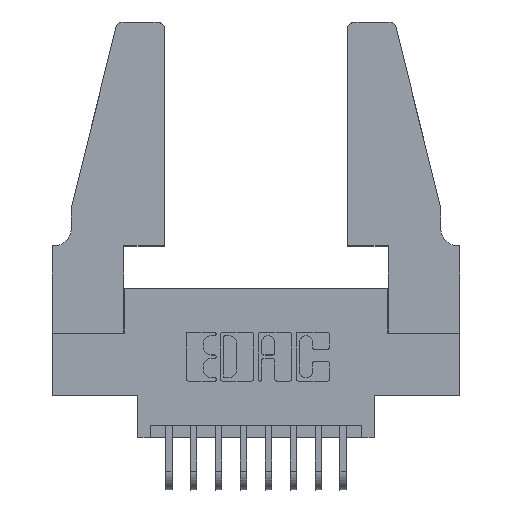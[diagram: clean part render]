
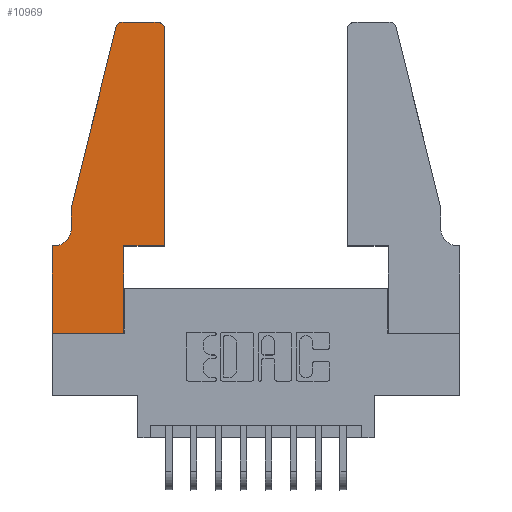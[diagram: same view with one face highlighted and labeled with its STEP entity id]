
A CAD part, top view. The second image highlights one B-rep face of the part: STEP entity #10969.
In plain terms, the highlighted planar face has unit normal (0, 0, 1).
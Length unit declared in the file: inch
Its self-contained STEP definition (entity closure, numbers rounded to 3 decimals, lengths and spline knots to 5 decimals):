
#28 = CARTESIAN_POINT ( 'NONE',  ( 0.25487, 1.22718, 0.37 ) ) ;
#66 = CARTESIAN_POINT ( 'NONE',  ( 0.2865, 0.35, 0.37 ) ) ;
#365 = LINE ( 'NONE', #3650, #8227 ) ;
#693 = VECTOR ( 'NONE', #12470, 39.37008 ) ;
#808 = ORIENTED_EDGE ( 'NONE', *, *, #6925, .T. ) ;
#941 = CARTESIAN_POINT ( 'NONE',  ( 0.4505, 0.35, 0.37 ) ) ;
#954 = ORIENTED_EDGE ( 'NONE', *, *, #7182, .T. ) ;
#988 = CARTESIAN_POINT ( 'NONE',  ( 0.2865, 0.35, 0.37 ) ) ;
#1146 = VERTEX_POINT ( 'NONE', #13948 ) ;
#1562 = ORIENTED_EDGE ( 'NONE', *, *, #14739, .T. ) ;
#1564 = LINE ( 'NONE', #11279, #4241 ) ;
#1579 = LINE ( 'NONE', #7947, #693 ) ;
#1586 = DIRECTION ( 'NONE',  ( 0., 0., 1. ) ) ;
#1688 = CARTESIAN_POINT ( 'NONE',  ( 0.4205, 1.22, 0.37 ) ) ;
#2029 = LINE ( 'NONE', #8240, #6129 ) ;
#2648 = EDGE_CURVE ( 'NONE', #11795, #11288, #12134, .T. ) ;
#2776 = EDGE_CURVE ( 'NONE', #5609, #3500, #8960, .T. ) ;
#3038 = FACE_OUTER_BOUND ( 'NONE', #5361, .T. ) ;
#3050 = DIRECTION ( 'NONE',  ( 0., 0., 1. ) ) ;
#3183 = EDGE_CURVE ( 'NONE', #1146, #6017, #3889, .T. ) ;
#3237 = EDGE_CURVE ( 'NONE', #3848, #1146, #1579, .T. ) ;
#3498 = DIRECTION ( 'NONE',  ( 0., 0., -1. ) ) ;
#3500 = VERTEX_POINT ( 'NONE', #6154 ) ;
#3650 = CARTESIAN_POINT ( 'NONE',  ( 0., 0., 0.37 ) ) ;
#3815 = ORIENTED_EDGE ( 'NONE', *, *, #7220, .T. ) ;
#3848 = VERTEX_POINT ( 'NONE', #3857 ) ;
#3857 = CARTESIAN_POINT ( 'NONE',  ( 0., 0., 0.37 ) ) ;
#3889 = LINE ( 'NONE', #988, #4594 ) ;
#4046 = PLANE ( 'NONE',  #5932 ) ;
#4065 = VERTEX_POINT ( 'NONE', #941 ) ;
#4241 = VECTOR ( 'NONE', #4418, 39.37008 ) ;
#4335 = AXIS2_PLACEMENT_3D ( 'NONE', #9169, #3498, #12606 ) ;
#4418 = DIRECTION ( 'NONE',  ( -1., 0., 0. ) ) ;
#4440 = ORIENTED_EDGE ( 'NONE', *, *, #3183, .T. ) ;
#4594 = VECTOR ( 'NONE', #6827, 39.37008 ) ;
#4680 = AXIS2_PLACEMENT_3D ( 'NONE', #1688, #1586, #14358 ) ;
#4840 = VECTOR ( 'NONE', #13643, 39.37008 ) ;
#5280 = DIRECTION ( 'NONE',  ( 1., 0., 0. ) ) ;
#5361 = EDGE_LOOP ( 'NONE', ( #3815, #8125, #5536, #9611, #8568, #6661, #1562, #12802, #4440, #13207, #954, #808 ) ) ;
#5536 = ORIENTED_EDGE ( 'NONE', *, *, #6741, .T. ) ;
#5609 = VERTEX_POINT ( 'NONE', #10730 ) ;
#5837 = VERTEX_POINT ( 'NONE', #13208 ) ;
#5872 = VECTOR ( 'NONE', #6796, 39.37008 ) ;
#5932 = AXIS2_PLACEMENT_3D ( 'NONE', #7614, #3050, #5280 ) ;
#6017 = VERTEX_POINT ( 'NONE', #66 ) ;
#6129 = VECTOR ( 'NONE', #9478, 39.37008 ) ;
#6154 = CARTESIAN_POINT ( 'NONE',  ( 0.0755, 0.42, 0.37 ) ) ;
#6302 = EDGE_CURVE ( 'NONE', #6017, #4065, #8851, .T. ) ;
#6324 = VECTOR ( 'NONE', #14458, 39.37008 ) ;
#6378 = CARTESIAN_POINT ( 'NONE',  ( 0.0755, 0.35, 0.37 ) ) ;
#6543 = CARTESIAN_POINT ( 'NONE',  ( 0.284, 1.22, 0.37 ) ) ;
#6596 = DIRECTION ( 'NONE',  ( 0., 0., 1. ) ) ;
#6661 = ORIENTED_EDGE ( 'NONE', *, *, #13215, .T. ) ;
#6741 = EDGE_CURVE ( 'NONE', #11288, #5609, #2029, .T. ) ;
#6796 = DIRECTION ( 'NONE',  ( 0., -1., 0. ) ) ;
#6827 = DIRECTION ( 'NONE',  ( 0., 1., 0. ) ) ;
#6925 = EDGE_CURVE ( 'NONE', #10156, #10413, #11331, .T. ) ;
#7182 = EDGE_CURVE ( 'NONE', #4065, #10156, #14001, .T. ) ;
#7220 = EDGE_CURVE ( 'NONE', #10413, #11795, #1564, .T. ) ;
#7614 = CARTESIAN_POINT ( 'NONE',  ( 0., 0.35, 0.37 ) ) ;
#7713 = DIRECTION ( 'NONE',  ( 1., 0., 0. ) ) ;
#7840 = CARTESIAN_POINT ( 'NONE',  ( 0.4505, 0.35, 0.37 ) ) ;
#7947 = CARTESIAN_POINT ( 'NONE',  ( 0., 0., 0.37 ) ) ;
#8125 = ORIENTED_EDGE ( 'NONE', *, *, #2648, .T. ) ;
#8227 = VECTOR ( 'NONE', #9466, 39.37008 ) ;
#8240 = CARTESIAN_POINT ( 'NONE',  ( 0.0755, 0.5, 0.37 ) ) ;
#8548 = VECTOR ( 'NONE', #9728, 39.37008 ) ;
#8568 = ORIENTED_EDGE ( 'NONE', *, *, #11293, .T. ) ;
#8851 = LINE ( 'NONE', #13198, #6324 ) ;
#8960 = LINE ( 'NONE', #10045, #5872 ) ;
#9169 = CARTESIAN_POINT ( 'NONE',  ( 0.0055, 0.42, 0.37 ) ) ;
#9466 = DIRECTION ( 'NONE',  ( 0., -1., 0. ) ) ;
#9478 = DIRECTION ( 'NONE',  ( -0.239, -0.971, 0. ) ) ;
#9611 = ORIENTED_EDGE ( 'NONE', *, *, #2776, .T. ) ;
#9728 = DIRECTION ( 'NONE',  ( -1., 0., 0. ) ) ;
#10045 = CARTESIAN_POINT ( 'NONE',  ( 0.0755, 0.5, 0.37 ) ) ;
#10156 = VERTEX_POINT ( 'NONE', #12154 ) ;
#10413 = VERTEX_POINT ( 'NONE', #11198 ) ;
#10697 = VERTEX_POINT ( 'NONE', #14632 ) ;
#10730 = CARTESIAN_POINT ( 'NONE',  ( 0.0755, 0.5, 0.37 ) ) ;
#10969 = ADVANCED_FACE ( 'NONE', ( #3038 ), #4046, .T. ) ;
#11198 = CARTESIAN_POINT ( 'NONE',  ( 0.4205, 1.25, 0.37 ) ) ;
#11279 = CARTESIAN_POINT ( 'NONE',  ( 0.2605, 1.25, 0.37 ) ) ;
#11288 = VERTEX_POINT ( 'NONE', #28 ) ;
#11293 = EDGE_CURVE ( 'NONE', #3500, #10697, #11978, .T. ) ;
#11331 = CIRCLE ( 'NONE', #4680, 0.03 ) ;
#11714 = AXIS2_PLACEMENT_3D ( 'NONE', #6543, #6596, #7713 ) ;
#11795 = VERTEX_POINT ( 'NONE', #13794 ) ;
#11978 = CIRCLE ( 'NONE', #4335, 0.07 ) ;
#12134 = CIRCLE ( 'NONE', #11714, 0.03 ) ;
#12154 = CARTESIAN_POINT ( 'NONE',  ( 0.4505, 1.22, 0.37 ) ) ;
#12470 = DIRECTION ( 'NONE',  ( 1., 0., 0. ) ) ;
#12606 = DIRECTION ( 'NONE',  ( -1., 0., 0. ) ) ;
#12802 = ORIENTED_EDGE ( 'NONE', *, *, #3237, .T. ) ;
#13198 = CARTESIAN_POINT ( 'NONE',  ( 0.4505, 0.35, 0.37 ) ) ;
#13207 = ORIENTED_EDGE ( 'NONE', *, *, #6302, .T. ) ;
#13208 = CARTESIAN_POINT ( 'NONE',  ( 0., 0.35, 0.37 ) ) ;
#13215 = EDGE_CURVE ( 'NONE', #10697, #5837, #13571, .T. ) ;
#13571 = LINE ( 'NONE', #6378, #8548 ) ;
#13643 = DIRECTION ( 'NONE',  ( 0., 1., 0. ) ) ;
#13794 = CARTESIAN_POINT ( 'NONE',  ( 0.284, 1.25, 0.37 ) ) ;
#13948 = CARTESIAN_POINT ( 'NONE',  ( 0.2865, 0., 0.37 ) ) ;
#14001 = LINE ( 'NONE', #7840, #4840 ) ;
#14358 = DIRECTION ( 'NONE',  ( 1., 0., 0. ) ) ;
#14458 = DIRECTION ( 'NONE',  ( 1., 0., 0. ) ) ;
#14632 = CARTESIAN_POINT ( 'NONE',  ( 0.0055, 0.35, 0.37 ) ) ;
#14739 = EDGE_CURVE ( 'NONE', #5837, #3848, #365, .T. ) ;
